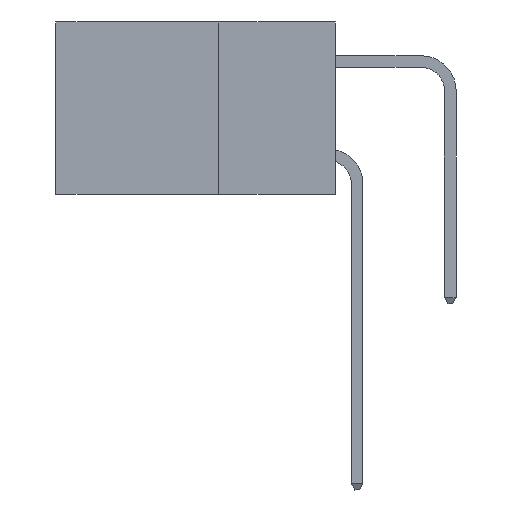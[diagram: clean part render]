
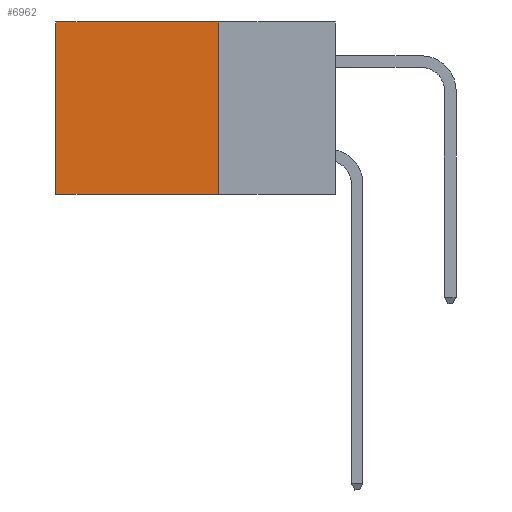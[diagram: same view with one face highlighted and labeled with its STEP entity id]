
A CAD part, left-side view. The second image highlights one B-rep face of the part: STEP entity #6962.
In plain terms, the highlighted planar face has unit normal (-1, 0, 0).
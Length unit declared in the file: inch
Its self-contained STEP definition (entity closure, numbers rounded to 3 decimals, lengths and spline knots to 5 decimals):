
#700 = LINE ( 'NONE', #12834, #4762 ) ;
#947 = ORIENTED_EDGE ( 'NONE', *, *, #9760, .F. ) ;
#1189 = CARTESIAN_POINT ( 'NONE',  ( 0.2875, 0.25, 0. ) ) ;
#3163 = LINE ( 'NONE', #3348, #10162 ) ;
#3348 = CARTESIAN_POINT ( 'NONE',  ( 0.2875, 0.6, 0. ) ) ;
#3792 = CARTESIAN_POINT ( 'NONE',  ( 0.2875, 0.25, -0.37 ) ) ;
#3879 = EDGE_CURVE ( 'NONE', #4547, #8772, #700, .T. ) ;
#4547 = VERTEX_POINT ( 'NONE', #14615 ) ;
#4702 = CARTESIAN_POINT ( 'NONE',  ( 0.2875, 0.6, -0.37 ) ) ;
#4762 = VECTOR ( 'NONE', #18698, 39.37008 ) ;
#5162 = LINE ( 'NONE', #20791, #11368 ) ;
#6108 = DIRECTION ( 'NONE',  ( 0., 1., 0. ) ) ;
#6454 = DIRECTION ( 'NONE',  ( 1., 0., 0. ) ) ;
#6962 = ADVANCED_FACE ( 'NONE', ( #15161 ), #18387, .F. ) ;
#6980 = DIRECTION ( 'NONE',  ( 0., 1., 0. ) ) ;
#7196 = EDGE_CURVE ( 'NONE', #10586, #22075, #3163, .T. ) ;
#8772 = VERTEX_POINT ( 'NONE', #3792 ) ;
#9760 = EDGE_CURVE ( 'NONE', #8772, #22075, #5162, .T. ) ;
#10136 = CARTESIAN_POINT ( 'NONE',  ( 0.2875, 0.25, 0. ) ) ;
#10162 = VECTOR ( 'NONE', #18733, 39.37008 ) ;
#10509 = LINE ( 'NONE', #1189, #19382 ) ;
#10586 = VERTEX_POINT ( 'NONE', #16670 ) ;
#11368 = VECTOR ( 'NONE', #6980, 39.37008 ) ;
#11702 = EDGE_CURVE ( 'NONE', #4547, #10586, #10509, .T. ) ;
#12834 = CARTESIAN_POINT ( 'NONE',  ( 0.2875, 0.25, 0. ) ) ;
#13452 = DIRECTION ( 'NONE',  ( 0., 0., -1. ) ) ;
#14579 = ORIENTED_EDGE ( 'NONE', *, *, #3879, .F. ) ;
#14615 = CARTESIAN_POINT ( 'NONE',  ( 0.2875, 0.25, 0. ) ) ;
#15161 = FACE_OUTER_BOUND ( 'NONE', #19926, .T. ) ;
#15943 = ORIENTED_EDGE ( 'NONE', *, *, #7196, .T. ) ;
#16670 = CARTESIAN_POINT ( 'NONE',  ( 0.2875, 0.6, 0. ) ) ;
#16966 = AXIS2_PLACEMENT_3D ( 'NONE', #10136, #6454, #13452 ) ;
#18387 = PLANE ( 'NONE',  #16966 ) ;
#18698 = DIRECTION ( 'NONE',  ( 0., 0., -1. ) ) ;
#18733 = DIRECTION ( 'NONE',  ( 0., 0., -1. ) ) ;
#19382 = VECTOR ( 'NONE', #6108, 39.37008 ) ;
#19542 = ORIENTED_EDGE ( 'NONE', *, *, #11702, .T. ) ;
#19926 = EDGE_LOOP ( 'NONE', ( #15943, #947, #14579, #19542 ) ) ;
#20791 = CARTESIAN_POINT ( 'NONE',  ( 0.2875, 0.25, -0.37 ) ) ;
#22075 = VERTEX_POINT ( 'NONE', #4702 ) ;
